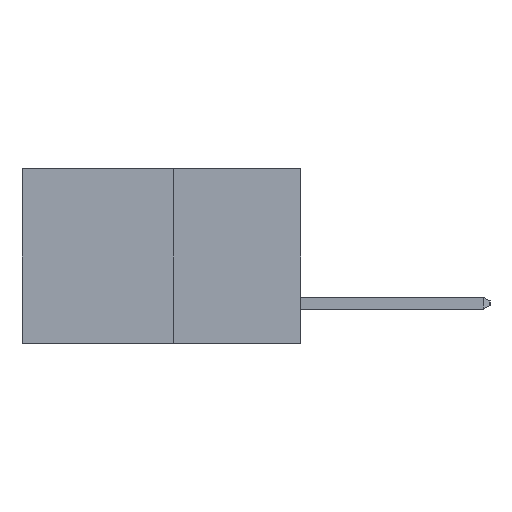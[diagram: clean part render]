
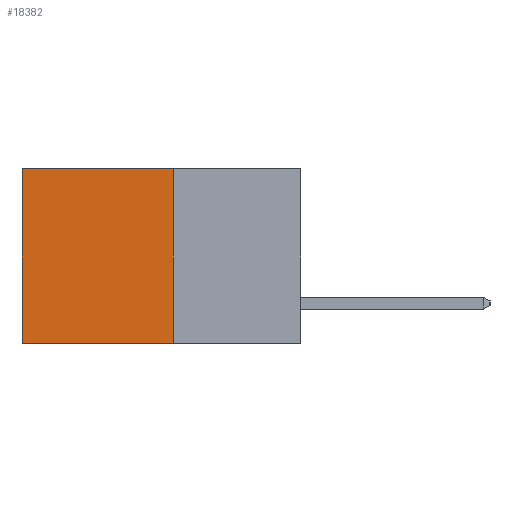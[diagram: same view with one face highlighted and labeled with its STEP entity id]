
A CAD part, left-side view. The second image highlights one B-rep face of the part: STEP entity #18382.
In plain terms, the highlighted planar face has unit normal (-1, 0, 0).
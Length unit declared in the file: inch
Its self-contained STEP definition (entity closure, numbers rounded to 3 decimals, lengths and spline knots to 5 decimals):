
#1711 = EDGE_CURVE ( 'NONE', #22516, #16568, #2277, .T. ) ;
#1722 = LINE ( 'NONE', #24460, #6549 ) ;
#1865 = EDGE_CURVE ( 'NONE', #16568, #9900, #14226, .T. ) ;
#2277 = LINE ( 'NONE', #23451, #12628 ) ;
#2436 = CARTESIAN_POINT ( 'NONE',  ( 0.277, 0.27, -0.37 ) ) ;
#2620 = CARTESIAN_POINT ( 'NONE',  ( 0.277, 0.59, 0. ) ) ;
#6414 = EDGE_CURVE ( 'NONE', #22516, #23695, #1722, .T. ) ;
#6549 = VECTOR ( 'NONE', #10195, 39.37008 ) ;
#6831 = CARTESIAN_POINT ( 'NONE',  ( 0.277, 0.27, 0. ) ) ;
#7128 = CARTESIAN_POINT ( 'NONE',  ( 0.277, 0.27, -0.37 ) ) ;
#9239 = DIRECTION ( 'NONE',  ( 0., 0., -1. ) ) ;
#9486 = FACE_OUTER_BOUND ( 'NONE', #22878, .T. ) ;
#9900 = VERTEX_POINT ( 'NONE', #26542 ) ;
#10195 = DIRECTION ( 'NONE',  ( 0., 0., -1. ) ) ;
#10832 = CARTESIAN_POINT ( 'NONE',  ( 0.277, 0.27, -0.37 ) ) ;
#11593 = ORIENTED_EDGE ( 'NONE', *, *, #1711, .T. ) ;
#12628 = VECTOR ( 'NONE', #25290, 39.37008 ) ;
#14226 = LINE ( 'NONE', #19285, #19014 ) ;
#14975 = DIRECTION ( 'NONE',  ( 0., 1., 0. ) ) ;
#15033 = VECTOR ( 'NONE', #14975, 39.37008 ) ;
#15878 = ORIENTED_EDGE ( 'NONE', *, *, #6414, .F. ) ;
#16568 = VERTEX_POINT ( 'NONE', #2620 ) ;
#17104 = EDGE_CURVE ( 'NONE', #23695, #9900, #21085, .T. ) ;
#17388 = PLANE ( 'NONE',  #17588 ) ;
#17588 = AXIS2_PLACEMENT_3D ( 'NONE', #7128, #21507, #9239 ) ;
#18382 = ADVANCED_FACE ( 'NONE', ( #9486 ), #17388, .F. ) ;
#19014 = VECTOR ( 'NONE', #26410, 39.37008 ) ;
#19285 = CARTESIAN_POINT ( 'NONE',  ( 0.277, 0.59, -0.37 ) ) ;
#21085 = LINE ( 'NONE', #10832, #15033 ) ;
#21507 = DIRECTION ( 'NONE',  ( 1., 0., 0. ) ) ;
#22516 = VERTEX_POINT ( 'NONE', #6831 ) ;
#22878 = EDGE_LOOP ( 'NONE', ( #25448, #23017, #15878, #11593 ) ) ;
#23017 = ORIENTED_EDGE ( 'NONE', *, *, #17104, .F. ) ;
#23451 = CARTESIAN_POINT ( 'NONE',  ( 0.277, 0.27, 0. ) ) ;
#23695 = VERTEX_POINT ( 'NONE', #2436 ) ;
#24460 = CARTESIAN_POINT ( 'NONE',  ( 0.277, 0.27, -0.37 ) ) ;
#25290 = DIRECTION ( 'NONE',  ( 0., 1., 0. ) ) ;
#25448 = ORIENTED_EDGE ( 'NONE', *, *, #1865, .T. ) ;
#26410 = DIRECTION ( 'NONE',  ( 0., 0., -1. ) ) ;
#26542 = CARTESIAN_POINT ( 'NONE',  ( 0.277, 0.59, -0.37 ) ) ;
